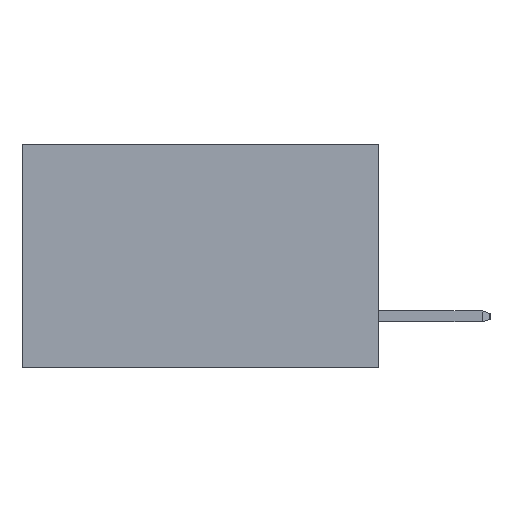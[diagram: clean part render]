
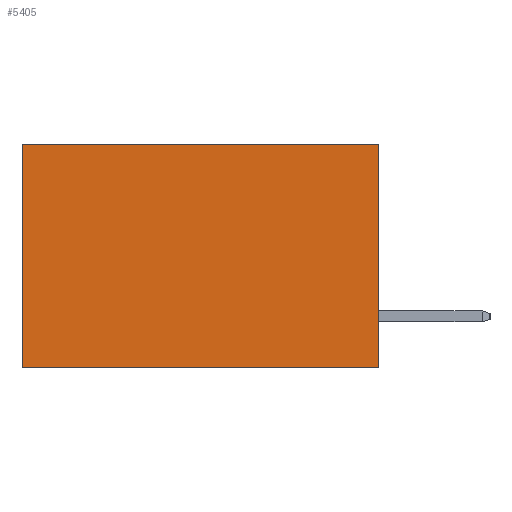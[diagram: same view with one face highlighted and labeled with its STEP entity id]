
A CAD part, left-side view. The second image highlights one B-rep face of the part: STEP entity #5405.
In plain terms, the highlighted planar face has unit normal (-1, 0, 0).
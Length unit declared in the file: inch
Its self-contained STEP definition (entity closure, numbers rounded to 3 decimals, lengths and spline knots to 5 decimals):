
#322 = LINE ( 'NONE', #4412, #23360 ) ;
#2330 = CARTESIAN_POINT ( 'NONE',  ( 0.277, 0., -0.37 ) ) ;
#3690 = ORIENTED_EDGE ( 'NONE', *, *, #21584, .T. ) ;
#4008 = CARTESIAN_POINT ( 'NONE',  ( 0.277, 0., -0.37 ) ) ;
#4251 = AXIS2_PLACEMENT_3D ( 'NONE', #8703, #5827, #5386 ) ;
#4412 = CARTESIAN_POINT ( 'NONE',  ( 0.277, 0., -0.37 ) ) ;
#5386 = DIRECTION ( 'NONE',  ( 0., 0., -1. ) ) ;
#5405 = ADVANCED_FACE ( 'NONE', ( #15606 ), #6518, .F. ) ;
#5827 = DIRECTION ( 'NONE',  ( 1., 0., 0. ) ) ;
#6518 = PLANE ( 'NONE',  #4251 ) ;
#7477 = DIRECTION ( 'NONE',  ( 0., 0., -1. ) ) ;
#7682 = DIRECTION ( 'NONE',  ( 0., 1., 0. ) ) ;
#8388 = CARTESIAN_POINT ( 'NONE',  ( 0.277, 0., 0. ) ) ;
#8703 = CARTESIAN_POINT ( 'NONE',  ( 0.277, 0., -0.37 ) ) ;
#8724 = CARTESIAN_POINT ( 'NONE',  ( 0.277, 0.59, 0. ) ) ;
#9116 = EDGE_CURVE ( 'NONE', #18805, #12526, #10869, .T. ) ;
#9275 = VECTOR ( 'NONE', #7682, 39.37008 ) ;
#9875 = ORIENTED_EDGE ( 'NONE', *, *, #9116, .F. ) ;
#10158 = VECTOR ( 'NONE', #15052, 39.37008 ) ;
#10604 = EDGE_CURVE ( 'NONE', #12526, #22063, #322, .T. ) ;
#10869 = LINE ( 'NONE', #4008, #10158 ) ;
#12526 = VERTEX_POINT ( 'NONE', #2330 ) ;
#14011 = EDGE_CURVE ( 'NONE', #20172, #22063, #23535, .T. ) ;
#14950 = ORIENTED_EDGE ( 'NONE', *, *, #14011, .T. ) ;
#15052 = DIRECTION ( 'NONE',  ( 0., 0., -1. ) ) ;
#15606 = FACE_OUTER_BOUND ( 'NONE', #25572, .T. ) ;
#18309 = VECTOR ( 'NONE', #7477, 39.37008 ) ;
#18703 = CARTESIAN_POINT ( 'NONE',  ( 0.277, 0., 0. ) ) ;
#18805 = VERTEX_POINT ( 'NONE', #8388 ) ;
#20172 = VERTEX_POINT ( 'NONE', #8724 ) ;
#21031 = LINE ( 'NONE', #18703, #9275 ) ;
#21584 = EDGE_CURVE ( 'NONE', #18805, #20172, #21031, .T. ) ;
#22063 = VERTEX_POINT ( 'NONE', #22554 ) ;
#22554 = CARTESIAN_POINT ( 'NONE',  ( 0.277, 0.59, -0.37 ) ) ;
#22959 = CARTESIAN_POINT ( 'NONE',  ( 0.277, 0.59, -0.37 ) ) ;
#23360 = VECTOR ( 'NONE', #28640, 39.37008 ) ;
#23535 = LINE ( 'NONE', #22959, #18309 ) ;
#25572 = EDGE_LOOP ( 'NONE', ( #14950, #28316, #9875, #3690 ) ) ;
#28316 = ORIENTED_EDGE ( 'NONE', *, *, #10604, .F. ) ;
#28640 = DIRECTION ( 'NONE',  ( 0., 1., 0. ) ) ;
